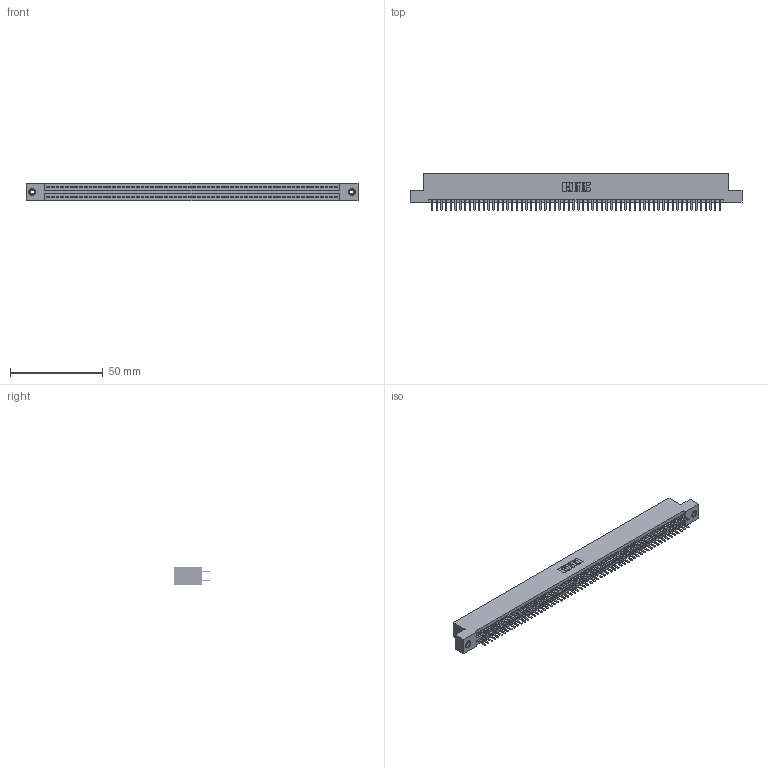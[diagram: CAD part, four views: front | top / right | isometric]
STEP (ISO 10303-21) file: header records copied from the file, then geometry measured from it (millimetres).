
FILE_DESCRIPTION (( 'STEP AP203' ), '1' );
FILE_NAME ('395-124-520-208.STEP', '2019-10-28T10:03:59', ( '' ), ( '' ), 'SwSTEP 2.0', 'SolidWorks 2016', '' );
FILE_SCHEMA (( 'CONFIG_CONTROL_DESIGN' ));
Length unit declared in the file: inch
Products named in the file (4): 395-124-520-208; 345 Part_Flush Mounting Lugs - 0.156 Dia-TI; 345-292-001_345-293-120; 345-250-001_345-250-003-102
Assembly tree (127 placements, depth 2):
  395-124-520-208
    345 Part_Flush Mounting Lugs - 0.156 Dia-TI
    345-292-001_345-293-120  x124
    345-250-001_345-250-003-102  x2
Bounding box: 178.69 x 19.68 x 9.4 mm (x, y, z)
Volume: 17482.6 mm3; surface area: 26127.1 mm2
Topology: 127 solids, 127 shells, 6882 faces, 19945 edges, 12958 vertices
Faces by surface type: plane 4452, cylinder 2414, cone 12, torus 4
Entity records: 47254 total; most frequent: CARTESIAN_POINT 7895, ORIENTED_EDGE 7810, DIRECTION 6951, EDGE_CURVE 3905, LINE 3501, VECTOR 3501, VERTEX_POINT 2596, AXIS2_PLACEMENT_3D 1725
